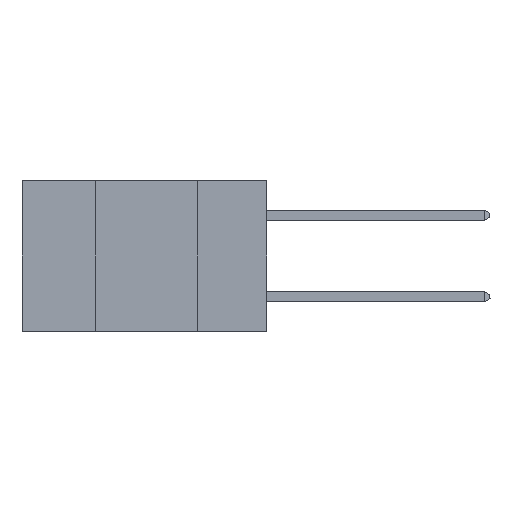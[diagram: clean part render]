
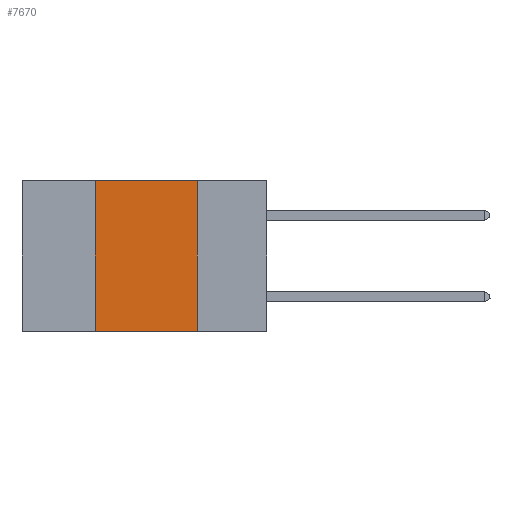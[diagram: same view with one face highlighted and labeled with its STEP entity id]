
A CAD part, left-side view. The second image highlights one B-rep face of the part: STEP entity #7670.
In plain terms, the highlighted planar face has unit normal (-1, 0, 0).
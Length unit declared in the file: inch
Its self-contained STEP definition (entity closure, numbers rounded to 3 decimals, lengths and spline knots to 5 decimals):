
#1969 = FACE_OUTER_BOUND ( 'NONE', #25308, .T. ) ;
#2833 = CARTESIAN_POINT ( 'NONE',  ( 0., 0.6, -0.37 ) ) ;
#2941 = EDGE_CURVE ( 'NONE', #7111, #19858, #5978, .T. ) ;
#3267 = DIRECTION ( 'NONE',  ( 0., 0., -1. ) ) ;
#3396 = CARTESIAN_POINT ( 'NONE',  ( 0., 0.6, 0. ) ) ;
#3895 = ORIENTED_EDGE ( 'NONE', *, *, #20316, .F. ) ;
#4137 = AXIS2_PLACEMENT_3D ( 'NONE', #21474, #17627, #8078 ) ;
#4540 = EDGE_CURVE ( 'NONE', #12812, #19858, #7680, .T. ) ;
#4553 = ORIENTED_EDGE ( 'NONE', *, *, #10718, .F. ) ;
#4877 = VECTOR ( 'NONE', #8216, 39.37008 ) ;
#5001 = CARTESIAN_POINT ( 'NONE',  ( 0., 0.17, 0. ) ) ;
#5606 = LINE ( 'NONE', #3396, #4877 ) ;
#5978 = LINE ( 'NONE', #5001, #19484 ) ;
#6517 = LINE ( 'NONE', #11034, #27530 ) ;
#7111 = VERTEX_POINT ( 'NONE', #20304 ) ;
#7670 = ADVANCED_FACE ( 'NONE', ( #1969 ), #11601, .F. ) ;
#7680 = LINE ( 'NONE', #2833, #26898 ) ;
#8078 = DIRECTION ( 'NONE',  ( 0., 0., -1. ) ) ;
#8216 = DIRECTION ( 'NONE',  ( 0., -1., 0. ) ) ;
#9914 = ORIENTED_EDGE ( 'NONE', *, *, #4540, .T. ) ;
#10718 = EDGE_CURVE ( 'NONE', #15594, #7111, #5606, .T. ) ;
#11034 = CARTESIAN_POINT ( 'NONE',  ( 0., 0.42, 0. ) ) ;
#11601 = PLANE ( 'NONE',  #4137 ) ;
#12812 = VERTEX_POINT ( 'NONE', #25031 ) ;
#15594 = VERTEX_POINT ( 'NONE', #27393 ) ;
#17394 = DIRECTION ( 'NONE',  ( 0., -1., 0. ) ) ;
#17627 = DIRECTION ( 'NONE',  ( 1., 0., 0. ) ) ;
#19484 = VECTOR ( 'NONE', #3267, 39.37008 ) ;
#19858 = VERTEX_POINT ( 'NONE', #27414 ) ;
#20304 = CARTESIAN_POINT ( 'NONE',  ( 0., 0.17, 0. ) ) ;
#20316 = EDGE_CURVE ( 'NONE', #12812, #15594, #6517, .T. ) ;
#21474 = CARTESIAN_POINT ( 'NONE',  ( 0., 0.6, 0. ) ) ;
#25031 = CARTESIAN_POINT ( 'NONE',  ( 0., 0.42, -0.37 ) ) ;
#25308 = EDGE_LOOP ( 'NONE', ( #30162, #4553, #3895, #9914 ) ) ;
#26898 = VECTOR ( 'NONE', #17394, 39.37008 ) ;
#27393 = CARTESIAN_POINT ( 'NONE',  ( 0., 0.42, 0. ) ) ;
#27414 = CARTESIAN_POINT ( 'NONE',  ( 0., 0.17, -0.37 ) ) ;
#27530 = VECTOR ( 'NONE', #27995, 39.37008 ) ;
#27995 = DIRECTION ( 'NONE',  ( 0., 0., 1. ) ) ;
#30162 = ORIENTED_EDGE ( 'NONE', *, *, #2941, .F. ) ;
